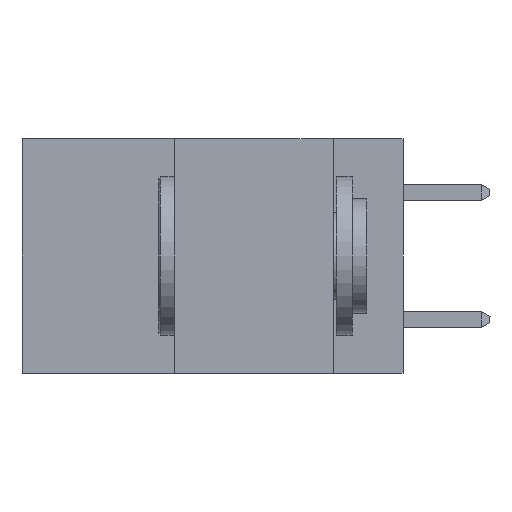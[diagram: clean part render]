
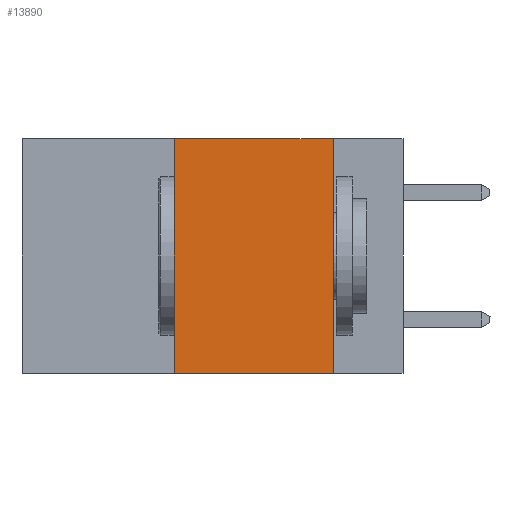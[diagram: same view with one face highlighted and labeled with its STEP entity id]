
A CAD part, left-side view. The second image highlights one B-rep face of the part: STEP entity #13890.
In plain terms, the highlighted planar face has unit normal (-1, 0, 0).
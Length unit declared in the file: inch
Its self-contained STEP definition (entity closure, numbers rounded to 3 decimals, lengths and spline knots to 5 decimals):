
#542 = VECTOR ( 'NONE', #2625, 39.37008 ) ;
#653 = VERTEX_POINT ( 'NONE', #16123 ) ;
#768 = CARTESIAN_POINT ( 'NONE',  ( 0., 0.11, 0. ) ) ;
#1365 = PLANE ( 'NONE',  #1713 ) ;
#1367 = DIRECTION ( 'NONE',  ( 0., -1., 0. ) ) ;
#1583 = DIRECTION ( 'NONE',  ( 0., 0., 1. ) ) ;
#1713 = AXIS2_PLACEMENT_3D ( 'NONE', #14863, #17987, #16384 ) ;
#1772 = ORIENTED_EDGE ( 'NONE', *, *, #15176, .F. ) ;
#2000 = EDGE_LOOP ( 'NONE', ( #1772, #14826, #13086, #16176 ) ) ;
#2625 = DIRECTION ( 'NONE',  ( 0., 0., -1. ) ) ;
#4008 = CARTESIAN_POINT ( 'NONE',  ( 0., 0.11, 0. ) ) ;
#5312 = VERTEX_POINT ( 'NONE', #768 ) ;
#6015 = VECTOR ( 'NONE', #1367, 39.37008 ) ;
#6067 = CARTESIAN_POINT ( 'NONE',  ( 0., 0.6, 0. ) ) ;
#6345 = VECTOR ( 'NONE', #1583, 39.37008 ) ;
#8949 = CARTESIAN_POINT ( 'NONE',  ( 0., 0.6, -0.37 ) ) ;
#9982 = VERTEX_POINT ( 'NONE', #10788 ) ;
#10559 = CARTESIAN_POINT ( 'NONE',  ( 0., 0.36, 0. ) ) ;
#10704 = LINE ( 'NONE', #8949, #6015 ) ;
#10788 = CARTESIAN_POINT ( 'NONE',  ( 0., 0.36, -0.37 ) ) ;
#11364 = VERTEX_POINT ( 'NONE', #16611 ) ;
#11367 = LINE ( 'NONE', #4008, #542 ) ;
#11521 = LINE ( 'NONE', #10559, #6345 ) ;
#13086 = ORIENTED_EDGE ( 'NONE', *, *, #16939, .F. ) ;
#13890 = ADVANCED_FACE ( 'NONE', ( #18720 ), #1365, .F. ) ;
#13986 = LINE ( 'NONE', #6067, #18190 ) ;
#14826 = ORIENTED_EDGE ( 'NONE', *, *, #15278, .F. ) ;
#14863 = CARTESIAN_POINT ( 'NONE',  ( 0., 0.6, 0. ) ) ;
#15176 = EDGE_CURVE ( 'NONE', #5312, #653, #11367, .T. ) ;
#15278 = EDGE_CURVE ( 'NONE', #11364, #5312, #13986, .T. ) ;
#15305 = DIRECTION ( 'NONE',  ( 0., -1., 0. ) ) ;
#16123 = CARTESIAN_POINT ( 'NONE',  ( 0., 0.11, -0.37 ) ) ;
#16176 = ORIENTED_EDGE ( 'NONE', *, *, #18570, .T. ) ;
#16384 = DIRECTION ( 'NONE',  ( 0., 0., -1. ) ) ;
#16611 = CARTESIAN_POINT ( 'NONE',  ( 0., 0.36, 0. ) ) ;
#16939 = EDGE_CURVE ( 'NONE', #9982, #11364, #11521, .T. ) ;
#17987 = DIRECTION ( 'NONE',  ( 1., 0., 0. ) ) ;
#18190 = VECTOR ( 'NONE', #15305, 39.37008 ) ;
#18570 = EDGE_CURVE ( 'NONE', #9982, #653, #10704, .T. ) ;
#18720 = FACE_OUTER_BOUND ( 'NONE', #2000, .T. ) ;
